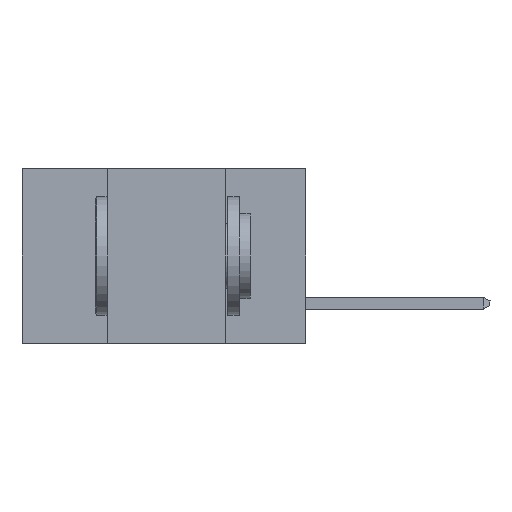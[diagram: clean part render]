
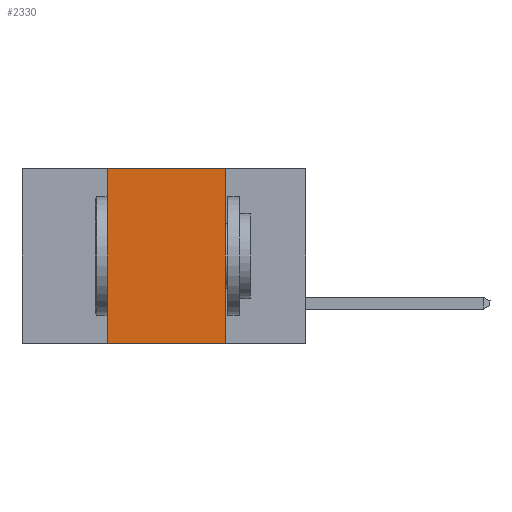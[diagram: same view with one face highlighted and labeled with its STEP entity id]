
A CAD part, left-side view. The second image highlights one B-rep face of the part: STEP entity #2330.
In plain terms, the highlighted planar face has unit normal (-1, 0, 0).
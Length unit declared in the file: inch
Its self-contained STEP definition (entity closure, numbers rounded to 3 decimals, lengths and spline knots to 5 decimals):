
#460 = VECTOR ( 'NONE', #3423, 39.37008 ) ;
#892 = CARTESIAN_POINT ( 'NONE',  ( 0., 0.6, 0. ) ) ;
#2121 = CARTESIAN_POINT ( 'NONE',  ( 0., 0.6, 0. ) ) ;
#2330 = ADVANCED_FACE ( 'NONE', ( #26353 ), #14327, .F. ) ;
#2521 = VECTOR ( 'NONE', #19357, 39.37008 ) ;
#3423 = DIRECTION ( 'NONE',  ( 0., 0., -1. ) ) ;
#4753 = LINE ( 'NONE', #892, #2521 ) ;
#5433 = EDGE_CURVE ( 'NONE', #11506, #5691, #14579, .T. ) ;
#5440 = CARTESIAN_POINT ( 'NONE',  ( 0., 0.17, 0. ) ) ;
#5691 = VERTEX_POINT ( 'NONE', #21948 ) ;
#6140 = DIRECTION ( 'NONE',  ( 1., 0., 0. ) ) ;
#8274 = LINE ( 'NONE', #22171, #10522 ) ;
#10159 = CARTESIAN_POINT ( 'NONE',  ( 0., 0.42, -0.37 ) ) ;
#10522 = VECTOR ( 'NONE', #20204, 39.37008 ) ;
#10981 = ORIENTED_EDGE ( 'NONE', *, *, #20565, .F. ) ;
#11506 = VERTEX_POINT ( 'NONE', #10159 ) ;
#12331 = CARTESIAN_POINT ( 'NONE',  ( 0., 0.6, -0.37 ) ) ;
#13055 = ORIENTED_EDGE ( 'NONE', *, *, #16470, .F. ) ;
#13628 = EDGE_CURVE ( 'NONE', #14321, #5691, #18659, .T. ) ;
#14250 = AXIS2_PLACEMENT_3D ( 'NONE', #2121, #6140, #22252 ) ;
#14321 = VERTEX_POINT ( 'NONE', #19168 ) ;
#14327 = PLANE ( 'NONE',  #14250 ) ;
#14579 = LINE ( 'NONE', #12331, #26489 ) ;
#16470 = EDGE_CURVE ( 'NONE', #11506, #17644, #8274, .T. ) ;
#17351 = ORIENTED_EDGE ( 'NONE', *, *, #5433, .T. ) ;
#17428 = ORIENTED_EDGE ( 'NONE', *, *, #13628, .F. ) ;
#17502 = EDGE_LOOP ( 'NONE', ( #17428, #10981, #13055, #17351 ) ) ;
#17644 = VERTEX_POINT ( 'NONE', #21385 ) ;
#18659 = LINE ( 'NONE', #5440, #460 ) ;
#19168 = CARTESIAN_POINT ( 'NONE',  ( 0., 0.17, 0. ) ) ;
#19357 = DIRECTION ( 'NONE',  ( 0., -1., 0. ) ) ;
#20204 = DIRECTION ( 'NONE',  ( 0., 0., 1. ) ) ;
#20505 = DIRECTION ( 'NONE',  ( 0., -1., 0. ) ) ;
#20565 = EDGE_CURVE ( 'NONE', #17644, #14321, #4753, .T. ) ;
#21385 = CARTESIAN_POINT ( 'NONE',  ( 0., 0.42, 0. ) ) ;
#21948 = CARTESIAN_POINT ( 'NONE',  ( 0., 0.17, -0.37 ) ) ;
#22171 = CARTESIAN_POINT ( 'NONE',  ( 0., 0.42, 0. ) ) ;
#22252 = DIRECTION ( 'NONE',  ( 0., 0., -1. ) ) ;
#26353 = FACE_OUTER_BOUND ( 'NONE', #17502, .T. ) ;
#26489 = VECTOR ( 'NONE', #20505, 39.37008 ) ;
